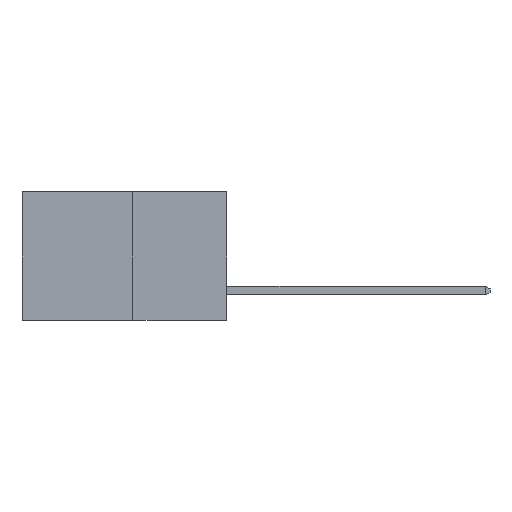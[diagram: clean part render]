
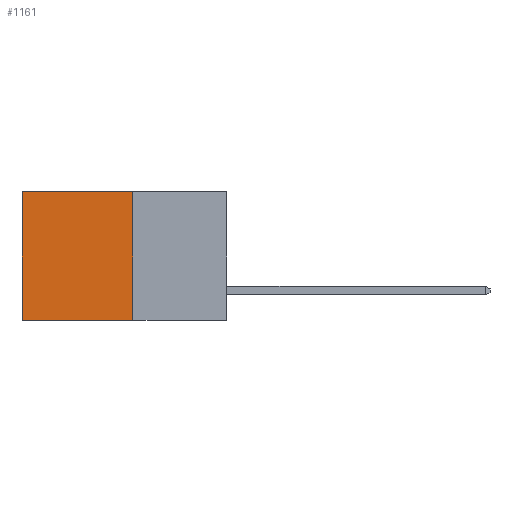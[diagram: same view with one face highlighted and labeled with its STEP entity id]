
A CAD part, left-side view. The second image highlights one B-rep face of the part: STEP entity #1161.
In plain terms, the highlighted planar face has unit normal (-1, 0, 0).
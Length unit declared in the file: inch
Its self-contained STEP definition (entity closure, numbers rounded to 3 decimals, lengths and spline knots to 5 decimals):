
#452 = LINE ( 'NONE', #500, #5532 ) ;
#500 = CARTESIAN_POINT ( 'NONE',  ( 0.277, 0.27, -0.37 ) ) ;
#522 = DIRECTION ( 'NONE',  ( 0., 1., 0. ) ) ;
#914 = FACE_OUTER_BOUND ( 'NONE', #1681, .T. ) ;
#1161 = ADVANCED_FACE ( 'NONE', ( #914 ), #9580, .F. ) ;
#1276 = CARTESIAN_POINT ( 'NONE',  ( 0.277, 0.27, 0. ) ) ;
#1616 = VECTOR ( 'NONE', #522, 39.37008 ) ;
#1681 = EDGE_LOOP ( 'NONE', ( #6850, #4486, #8723, #3841 ) ) ;
#1878 = LINE ( 'NONE', #10814, #1616 ) ;
#2379 = VECTOR ( 'NONE', #5819, 39.37008 ) ;
#3439 = CARTESIAN_POINT ( 'NONE',  ( 0.277, 0.27, -0.37 ) ) ;
#3648 = CARTESIAN_POINT ( 'NONE',  ( 0.277, 0.27, -0.37 ) ) ;
#3841 = ORIENTED_EDGE ( 'NONE', *, *, #8626, .T. ) ;
#4035 = VERTEX_POINT ( 'NONE', #7703 ) ;
#4397 = LINE ( 'NONE', #4955, #2379 ) ;
#4486 = ORIENTED_EDGE ( 'NONE', *, *, #7285, .F. ) ;
#4873 = VERTEX_POINT ( 'NONE', #4967 ) ;
#4955 = CARTESIAN_POINT ( 'NONE',  ( 0.277, 0.59, -0.37 ) ) ;
#4967 = CARTESIAN_POINT ( 'NONE',  ( 0.277, 0.27, 0. ) ) ;
#5305 = DIRECTION ( 'NONE',  ( 0., 0., -1. ) ) ;
#5532 = VECTOR ( 'NONE', #9913, 39.37008 ) ;
#5819 = DIRECTION ( 'NONE',  ( 0., 0., -1. ) ) ;
#6379 = VERTEX_POINT ( 'NONE', #7840 ) ;
#6652 = EDGE_CURVE ( 'NONE', #4873, #9339, #452, .T. ) ;
#6850 = ORIENTED_EDGE ( 'NONE', *, *, #9051, .T. ) ;
#7191 = AXIS2_PLACEMENT_3D ( 'NONE', #3439, #10469, #5305 ) ;
#7264 = DIRECTION ( 'NONE',  ( 0., 1., 0. ) ) ;
#7285 = EDGE_CURVE ( 'NONE', #9339, #6379, #1878, .T. ) ;
#7703 = CARTESIAN_POINT ( 'NONE',  ( 0.277, 0.59, 0. ) ) ;
#7840 = CARTESIAN_POINT ( 'NONE',  ( 0.277, 0.59, -0.37 ) ) ;
#8433 = VECTOR ( 'NONE', #7264, 39.37008 ) ;
#8626 = EDGE_CURVE ( 'NONE', #4873, #4035, #10466, .T. ) ;
#8723 = ORIENTED_EDGE ( 'NONE', *, *, #6652, .F. ) ;
#9051 = EDGE_CURVE ( 'NONE', #4035, #6379, #4397, .T. ) ;
#9339 = VERTEX_POINT ( 'NONE', #3648 ) ;
#9580 = PLANE ( 'NONE',  #7191 ) ;
#9913 = DIRECTION ( 'NONE',  ( 0., 0., -1. ) ) ;
#10466 = LINE ( 'NONE', #1276, #8433 ) ;
#10469 = DIRECTION ( 'NONE',  ( 1., 0., 0. ) ) ;
#10814 = CARTESIAN_POINT ( 'NONE',  ( 0.277, 0.27, -0.37 ) ) ;
